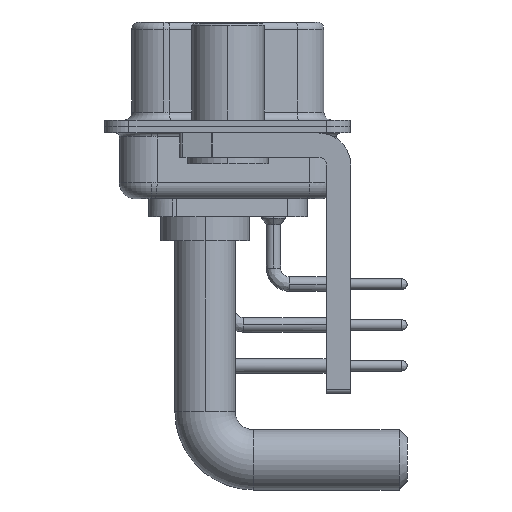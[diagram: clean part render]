
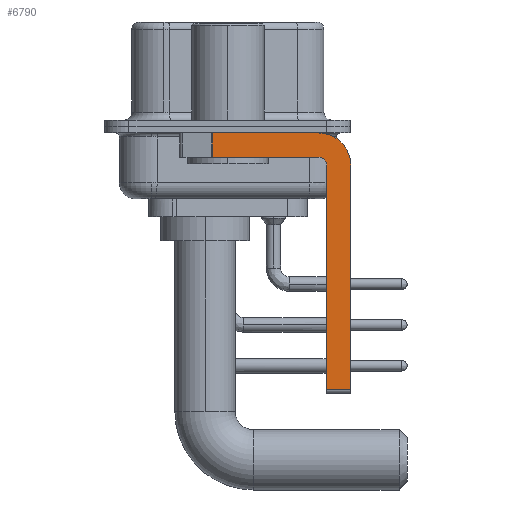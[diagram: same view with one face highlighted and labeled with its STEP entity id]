
A CAD part, left-side view. The second image highlights one B-rep face of the part: STEP entity #6790.
In plain terms, the highlighted planar face has unit normal (-1, 0, 0).
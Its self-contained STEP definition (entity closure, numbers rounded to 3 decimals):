
#115 = VERTEX_POINT ( 'NONE', #36611 ) ;
#276 = EDGE_CURVE ( 'NONE', #115, #22110, #14668, .T. ) ;
#402 = VECTOR ( 'NONE', #25193, 1000. ) ;
#474 = CARTESIAN_POINT ( 'NONE',  ( -2.9, -5.65, -0.4 ) ) ;
#1614 = DIRECTION ( 'NONE',  ( 0., 0., 1. ) ) ;
#2406 = CARTESIAN_POINT ( 'NONE',  ( -2.9, -5.65, -2.4 ) ) ;
#4558 = DIRECTION ( 'NONE',  ( 0., 0., -1. ) ) ;
#5329 = CARTESIAN_POINT ( 'NONE',  ( -2.9, -5.65, -1.9 ) ) ;
#5405 = VERTEX_POINT ( 'NONE', #474 ) ;
#5592 = VERTEX_POINT ( 'NONE', #9076 ) ;
#5974 = VERTEX_POINT ( 'NONE', #34100 ) ;
#6790 = ADVANCED_FACE ( 'NONE', ( #24746 ), #18794, .F. ) ;
#7464 = AXIS2_PLACEMENT_3D ( 'NONE', #32685, #21899, #1614 ) ;
#7607 = LINE ( 'NONE', #18948, #10894 ) ;
#7809 = DIRECTION ( 'NONE',  ( 0., 0., -1. ) ) ;
#7899 = LINE ( 'NONE', #13830, #402 ) ;
#8292 = VECTOR ( 'NONE', #19631, 1000. ) ;
#8949 = CARTESIAN_POINT ( 'NONE',  ( -2.9, -7.65, -16.35 ) ) ;
#9076 = CARTESIAN_POINT ( 'NONE',  ( -2.9, 0.978, -0.4 ) ) ;
#9973 = EDGE_CURVE ( 'NONE', #31537, #22110, #7607, .T. ) ;
#9986 = CARTESIAN_POINT ( 'NONE',  ( -2.9, 3., -0.4 ) ) ;
#10161 = DIRECTION ( 'NONE',  ( 0., -1., 0. ) ) ;
#10894 = VECTOR ( 'NONE', #33814, 1000. ) ;
#11754 = EDGE_CURVE ( 'NONE', #23720, #22215, #27660, .T. ) ;
#12388 = CARTESIAN_POINT ( 'NONE',  ( -2.9, 0.978, -1.9 ) ) ;
#12548 = EDGE_CURVE ( 'NONE', #5592, #5405, #18368, .T. ) ;
#13120 = EDGE_CURVE ( 'NONE', #115, #23720, #7899, .T. ) ;
#13213 = CARTESIAN_POINT ( 'NONE',  ( -2.9, -5.65, -1.9 ) ) ;
#13228 = ORIENTED_EDGE ( 'NONE', *, *, #12548, .F. ) ;
#13654 = CIRCLE ( 'NONE', #27931, 2. ) ;
#13830 = CARTESIAN_POINT ( 'NONE',  ( -2.9, -6.15, -16.6 ) ) ;
#14668 = LINE ( 'NONE', #23050, #23771 ) ;
#14918 = ORIENTED_EDGE ( 'NONE', *, *, #276, .T. ) ;
#16289 = EDGE_CURVE ( 'NONE', #5592, #5974, #35060, .T. ) ;
#17386 = EDGE_CURVE ( 'NONE', #22215, #5974, #27843, .T. ) ;
#17500 = ORIENTED_EDGE ( 'NONE', *, *, #17386, .F. ) ;
#17579 = VECTOR ( 'NONE', #10161, 1000. ) ;
#17599 = DIRECTION ( 'NONE',  ( 0., 0., -1. ) ) ;
#17825 = EDGE_CURVE ( 'NONE', #5405, #31537, #13654, .T. ) ;
#18368 = LINE ( 'NONE', #9986, #17579 ) ;
#18794 = PLANE ( 'NONE',  #26228 ) ;
#18948 = CARTESIAN_POINT ( 'NONE',  ( -2.9, -7.65, -2.4 ) ) ;
#19631 = DIRECTION ( 'NONE',  ( 0., 1., 0. ) ) ;
#19647 = CARTESIAN_POINT ( 'NONE',  ( -2.9, -7.65, -2.4 ) ) ;
#19945 = ORIENTED_EDGE ( 'NONE', *, *, #16289, .T. ) ;
#20078 = CARTESIAN_POINT ( 'NONE',  ( -2.9, -6.15, -2.4 ) ) ;
#20245 = EDGE_LOOP ( 'NONE', ( #13228, #19945, #17500, #24789, #32643, #14918, #32600, #27377 ) ) ;
#21899 = DIRECTION ( 'NONE',  ( -1., 0., 0. ) ) ;
#22110 = VERTEX_POINT ( 'NONE', #8949 ) ;
#22215 = VERTEX_POINT ( 'NONE', #13213 ) ;
#23050 = CARTESIAN_POINT ( 'NONE',  ( -2.9, -5.65, -16.35 ) ) ;
#23720 = VERTEX_POINT ( 'NONE', #20078 ) ;
#23771 = VECTOR ( 'NONE', #34741, 1000. ) ;
#24430 = CARTESIAN_POINT ( 'NONE',  ( -2.9, -5.65, -2.4 ) ) ;
#24551 = DIRECTION ( 'NONE',  ( 1., 0., 0. ) ) ;
#24746 = FACE_OUTER_BOUND ( 'NONE', #20245, .T. ) ;
#24789 = ORIENTED_EDGE ( 'NONE', *, *, #11754, .F. ) ;
#25193 = DIRECTION ( 'NONE',  ( 0., 0., 1. ) ) ;
#26228 = AXIS2_PLACEMENT_3D ( 'NONE', #2406, #24551, #7809 ) ;
#27377 = ORIENTED_EDGE ( 'NONE', *, *, #17825, .F. ) ;
#27660 = CIRCLE ( 'NONE', #7464, 0.5 ) ;
#27843 = LINE ( 'NONE', #5329, #8292 ) ;
#27931 = AXIS2_PLACEMENT_3D ( 'NONE', #24430, #32810, #4558 ) ;
#30226 = VECTOR ( 'NONE', #17599, 1000. ) ;
#31537 = VERTEX_POINT ( 'NONE', #19647 ) ;
#32600 = ORIENTED_EDGE ( 'NONE', *, *, #9973, .F. ) ;
#32643 = ORIENTED_EDGE ( 'NONE', *, *, #13120, .F. ) ;
#32685 = CARTESIAN_POINT ( 'NONE',  ( -2.9, -5.65, -2.4 ) ) ;
#32810 = DIRECTION ( 'NONE',  ( 1., 0., 0. ) ) ;
#33814 = DIRECTION ( 'NONE',  ( 0., 0., -1. ) ) ;
#34100 = CARTESIAN_POINT ( 'NONE',  ( -2.9, 0.978, -1.9 ) ) ;
#34741 = DIRECTION ( 'NONE',  ( 0., -1., 0. ) ) ;
#35060 = LINE ( 'NONE', #12388, #30226 ) ;
#36611 = CARTESIAN_POINT ( 'NONE',  ( -2.9, -6.15, -16.35 ) ) ;
